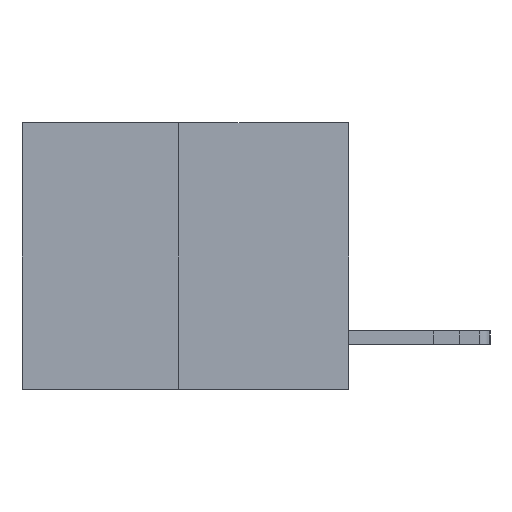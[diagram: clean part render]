
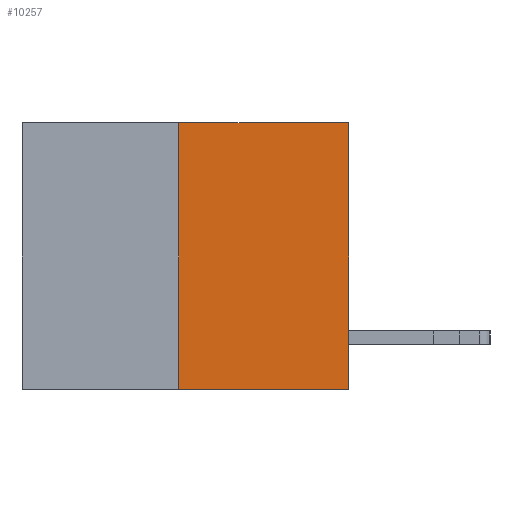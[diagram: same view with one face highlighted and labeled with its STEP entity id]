
A CAD part, left-side view. The second image highlights one B-rep face of the part: STEP entity #10257.
In plain terms, the highlighted planar face has unit normal (-1, 0, 0).
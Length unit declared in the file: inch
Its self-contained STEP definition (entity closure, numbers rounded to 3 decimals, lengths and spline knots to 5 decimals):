
#827 = DIRECTION ( 'NONE',  ( 0., -1., 0. ) ) ;
#1003 = VERTEX_POINT ( 'NONE', #22250 ) ;
#1351 = DIRECTION ( 'NONE',  ( 0., 0., -1. ) ) ;
#5063 = CARTESIAN_POINT ( 'NONE',  ( 0., 0.6, 0. ) ) ;
#5285 = CARTESIAN_POINT ( 'NONE',  ( 0., 0., 0. ) ) ;
#5794 = EDGE_CURVE ( 'NONE', #17057, #6205, #21413, .T. ) ;
#5870 = VECTOR ( 'NONE', #21574, 39.37008 ) ;
#6056 = EDGE_CURVE ( 'NONE', #1003, #8928, #6518, .T. ) ;
#6205 = VERTEX_POINT ( 'NONE', #17356 ) ;
#6518 = LINE ( 'NONE', #13774, #19555 ) ;
#8001 = AXIS2_PLACEMENT_3D ( 'NONE', #17705, #19538, #1351 ) ;
#8831 = EDGE_CURVE ( 'NONE', #17057, #1003, #15605, .T. ) ;
#8923 = FACE_OUTER_BOUND ( 'NONE', #25976, .T. ) ;
#8928 = VERTEX_POINT ( 'NONE', #5285 ) ;
#10257 = ADVANCED_FACE ( 'NONE', ( #8923 ), #21709, .F. ) ;
#10682 = ORIENTED_EDGE ( 'NONE', *, *, #17558, .F. ) ;
#11870 = ORIENTED_EDGE ( 'NONE', *, *, #8831, .T. ) ;
#13689 = DIRECTION ( 'NONE',  ( 0., 0., 1. ) ) ;
#13774 = CARTESIAN_POINT ( 'NONE',  ( 0., 0., 0. ) ) ;
#15605 = LINE ( 'NONE', #25340, #20650 ) ;
#17057 = VERTEX_POINT ( 'NONE', #25064 ) ;
#17063 = DIRECTION ( 'NONE',  ( 0., -1., 0. ) ) ;
#17356 = CARTESIAN_POINT ( 'NONE',  ( 0., 0.312, 0. ) ) ;
#17558 = EDGE_CURVE ( 'NONE', #6205, #8928, #25320, .T. ) ;
#17705 = CARTESIAN_POINT ( 'NONE',  ( 0., 0.6, 0. ) ) ;
#18841 = ORIENTED_EDGE ( 'NONE', *, *, #6056, .T. ) ;
#19538 = DIRECTION ( 'NONE',  ( 1., 0., 0. ) ) ;
#19555 = VECTOR ( 'NONE', #13689, 39.37008 ) ;
#20650 = VECTOR ( 'NONE', #17063, 39.37008 ) ;
#21413 = LINE ( 'NONE', #23719, #5870 ) ;
#21574 = DIRECTION ( 'NONE',  ( 0., 0., 1. ) ) ;
#21709 = PLANE ( 'NONE',  #8001 ) ;
#22250 = CARTESIAN_POINT ( 'NONE',  ( 0., 0., -0.49 ) ) ;
#22496 = VECTOR ( 'NONE', #827, 39.37008 ) ;
#23719 = CARTESIAN_POINT ( 'NONE',  ( 0., 0.312, -0.49 ) ) ;
#25064 = CARTESIAN_POINT ( 'NONE',  ( 0., 0.312, -0.49 ) ) ;
#25320 = LINE ( 'NONE', #5063, #22496 ) ;
#25340 = CARTESIAN_POINT ( 'NONE',  ( 0., 0.6, -0.49 ) ) ;
#25964 = ORIENTED_EDGE ( 'NONE', *, *, #5794, .F. ) ;
#25976 = EDGE_LOOP ( 'NONE', ( #25964, #11870, #18841, #10682 ) ) ;
